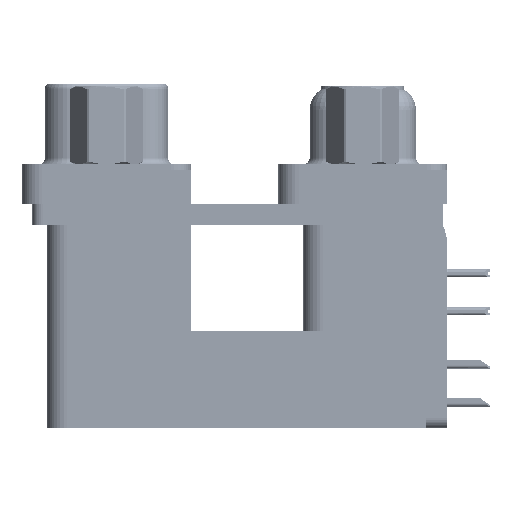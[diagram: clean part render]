
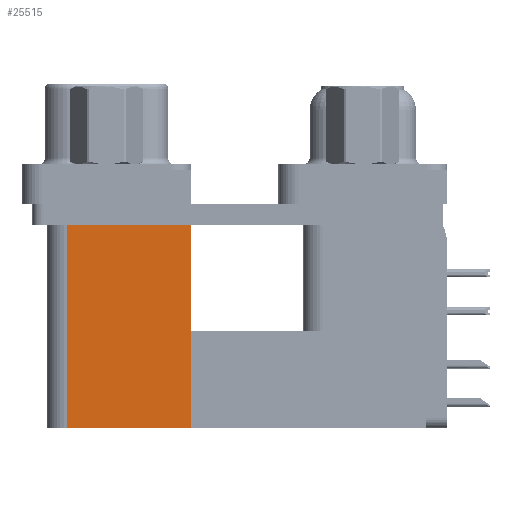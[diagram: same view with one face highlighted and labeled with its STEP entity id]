
A CAD part, left-side view. The second image highlights one B-rep face of the part: STEP entity #25515.
In plain terms, the highlighted planar face has unit normal (-1, 0, 0).
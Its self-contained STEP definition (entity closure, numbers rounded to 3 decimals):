
#161 = CARTESIAN_POINT ( 'NONE',  ( 3.7, 12.775, -2.5 ) ) ;
#3986 = ORIENTED_EDGE ( 'NONE', *, *, #55249, .F. ) ;
#4611 = VERTEX_POINT ( 'NONE', #11032 ) ;
#6223 = PLANE ( 'NONE',  #49966 ) ;
#6819 = DIRECTION ( 'NONE',  ( 0., 1., 0. ) ) ;
#9175 = CARTESIAN_POINT ( 'NONE',  ( 3.7, 21.975, -19.2 ) ) ;
#11032 = CARTESIAN_POINT ( 'NONE',  ( 3.7, 21.975, -2.5 ) ) ;
#12184 = VERTEX_POINT ( 'NONE', #50276 ) ;
#12413 = EDGE_CURVE ( 'NONE', #12184, #22946, #25168, .T. ) ;
#12706 = VECTOR ( 'NONE', #42033, 1000. ) ;
#12832 = VECTOR ( 'NONE', #13725, 1000. ) ;
#13725 = DIRECTION ( 'NONE',  ( 0., 0., 1. ) ) ;
#14740 = LINE ( 'NONE', #51885, #44766 ) ;
#22946 = VERTEX_POINT ( 'NONE', #161 ) ;
#25168 = LINE ( 'NONE', #33919, #26387 ) ;
#25515 = ADVANCED_FACE ( 'NONE', ( #38206 ), #6223, .F. ) ;
#26287 = ORIENTED_EDGE ( 'NONE', *, *, #50651, .T. ) ;
#26387 = VECTOR ( 'NONE', #53540, 1000. ) ;
#28121 = LINE ( 'NONE', #37476, #12706 ) ;
#29228 = DIRECTION ( 'NONE',  ( 0., 1., 0. ) ) ;
#30050 = CARTESIAN_POINT ( 'NONE',  ( 3.7, 12.775, -19.2 ) ) ;
#30240 = ORIENTED_EDGE ( 'NONE', *, *, #33877, .F. ) ;
#33877 = EDGE_CURVE ( 'NONE', #58149, #4611, #54506, .T. ) ;
#33919 = CARTESIAN_POINT ( 'NONE',  ( 3.7, 12.775, -19.2 ) ) ;
#37476 = CARTESIAN_POINT ( 'NONE',  ( 3.7, 12.775, -2.5 ) ) ;
#38206 = FACE_OUTER_BOUND ( 'NONE', #54937, .T. ) ;
#41780 = ORIENTED_EDGE ( 'NONE', *, *, #12413, .T. ) ;
#42033 = DIRECTION ( 'NONE',  ( 0., 1., 0. ) ) ;
#43942 = DIRECTION ( 'NONE',  ( 1., 0., 0. ) ) ;
#44766 = VECTOR ( 'NONE', #29228, 1000. ) ;
#49131 = CARTESIAN_POINT ( 'NONE',  ( 3.7, 21.975, -19.2 ) ) ;
#49966 = AXIS2_PLACEMENT_3D ( 'NONE', #30050, #43942, #6819 ) ;
#50276 = CARTESIAN_POINT ( 'NONE',  ( 3.7, 12.775, -19.2 ) ) ;
#50651 = EDGE_CURVE ( 'NONE', #22946, #4611, #28121, .T. ) ;
#51885 = CARTESIAN_POINT ( 'NONE',  ( 3.7, 12.775, -19.2 ) ) ;
#53540 = DIRECTION ( 'NONE',  ( 0., 0., 1. ) ) ;
#54506 = LINE ( 'NONE', #9175, #12832 ) ;
#54937 = EDGE_LOOP ( 'NONE', ( #26287, #30240, #3986, #41780 ) ) ;
#55249 = EDGE_CURVE ( 'NONE', #12184, #58149, #14740, .T. ) ;
#58149 = VERTEX_POINT ( 'NONE', #49131 ) ;
